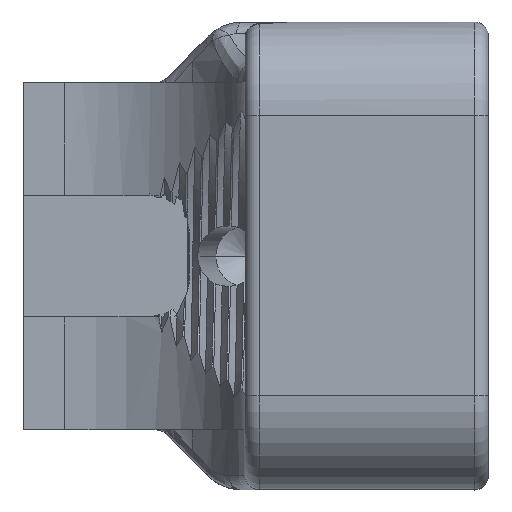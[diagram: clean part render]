
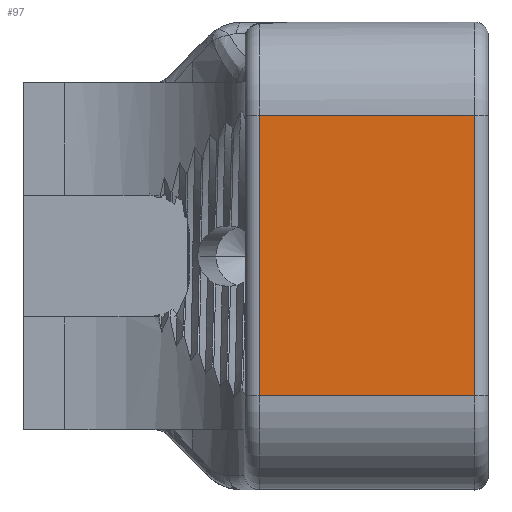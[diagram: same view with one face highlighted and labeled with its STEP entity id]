
A CAD part, top view. The second image highlights one B-rep face of the part: STEP entity #97.
In plain terms, the highlighted planar face has unit normal (0, 0, 1).
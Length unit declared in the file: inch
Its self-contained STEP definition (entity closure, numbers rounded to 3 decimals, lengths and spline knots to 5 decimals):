
#97 = ADVANCED_FACE ( 'NONE', ( #18370 ), #15607, .T. ) ;
#594 = AXIS2_PLACEMENT_3D ( 'NONE', #15954, #9512, #8680 ) ;
#1838 = CARTESIAN_POINT ( 'NONE',  ( 3.77818, 0.59055, 0.06777 ) ) ;
#2146 = VERTEX_POINT ( 'NONE', #17726 ) ;
#2180 = VECTOR ( 'NONE', #3086, 39.37008 ) ;
#2247 = LINE ( 'NONE', #3241, #2180 ) ;
#2647 = CARTESIAN_POINT ( 'NONE',  ( 3.77818, -0.59055, 0.06777 ) ) ;
#2907 = EDGE_LOOP ( 'NONE', ( #17236, #17273, #17294, #17310 ) ) ;
#3086 = DIRECTION ( 'NONE',  ( 0., 1., 0. ) ) ;
#3231 = LINE ( 'NONE', #8957, #3619 ) ;
#3241 = CARTESIAN_POINT ( 'NONE',  ( 4.68369, 0.98425, 0.06777 ) ) ;
#3541 = VERTEX_POINT ( 'NONE', #10740 ) ;
#3619 = VECTOR ( 'NONE', #8918, 39.37008 ) ;
#5602 = EDGE_CURVE ( 'NONE', #6638, #3541, #3231, .T. ) ;
#6352 = EDGE_CURVE ( 'NONE', #2146, #3541, #2247, .T. ) ;
#6638 = VERTEX_POINT ( 'NONE', #1838 ) ;
#7916 = VECTOR ( 'NONE', #13255, 39.37008 ) ;
#8191 = LINE ( 'NONE', #13324, #7916 ) ;
#8530 = EDGE_CURVE ( 'NONE', #6638, #14165, #19032, .T. ) ;
#8680 = DIRECTION ( 'NONE',  ( 1., 0., 0. ) ) ;
#8714 = DIRECTION ( 'NONE',  ( 0., -1., 0. ) ) ;
#8918 = DIRECTION ( 'NONE',  ( 1., 0., 0. ) ) ;
#8957 = CARTESIAN_POINT ( 'NONE',  ( 4.21228, 0.59055, 0.06777 ) ) ;
#9512 = DIRECTION ( 'NONE',  ( 0., 0., 1. ) ) ;
#10740 = CARTESIAN_POINT ( 'NONE',  ( 4.68369, 0.59055, 0.06777 ) ) ;
#10966 = CARTESIAN_POINT ( 'NONE',  ( 3.77818, -0.59055, 0.06777 ) ) ;
#13255 = DIRECTION ( 'NONE',  ( 1., 0., 0. ) ) ;
#13324 = CARTESIAN_POINT ( 'NONE',  ( 4.21228, -0.59055, 0.06777 ) ) ;
#14165 = VERTEX_POINT ( 'NONE', #2647 ) ;
#15607 = PLANE ( 'NONE',  #594 ) ;
#15954 = CARTESIAN_POINT ( 'NONE',  ( 4.21228, 0.98425, 0.06777 ) ) ;
#17236 = ORIENTED_EDGE ( 'NONE', *, *, #5602, .F. ) ;
#17273 = ORIENTED_EDGE ( 'NONE', *, *, #8530, .T. ) ;
#17294 = ORIENTED_EDGE ( 'NONE', *, *, #19076, .T. ) ;
#17310 = ORIENTED_EDGE ( 'NONE', *, *, #6352, .T. ) ;
#17726 = CARTESIAN_POINT ( 'NONE',  ( 4.68369, -0.59055, 0.06777 ) ) ;
#18370 = FACE_OUTER_BOUND ( 'NONE', #2907, .T. ) ;
#18978 = VECTOR ( 'NONE', #8714, 39.37008 ) ;
#19032 = LINE ( 'NONE', #10966, #18978 ) ;
#19076 = EDGE_CURVE ( 'NONE', #14165, #2146, #8191, .T. ) ;
